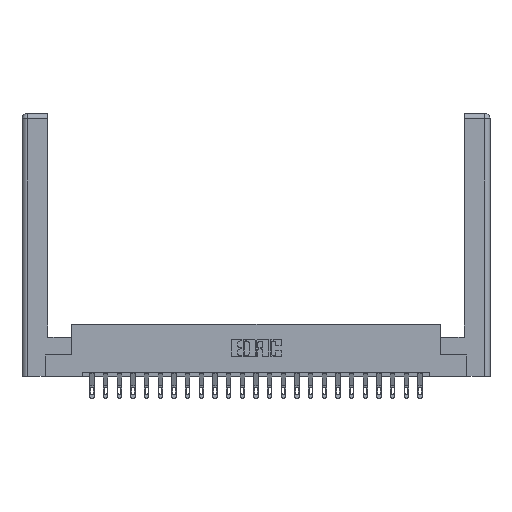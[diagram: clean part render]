
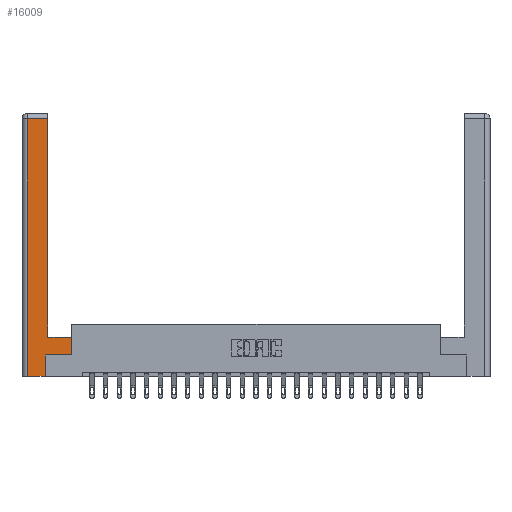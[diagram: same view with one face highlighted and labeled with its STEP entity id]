
A CAD part, top view. The second image highlights one B-rep face of the part: STEP entity #16009.
In plain terms, the highlighted planar face has unit normal (0, 0, 1).
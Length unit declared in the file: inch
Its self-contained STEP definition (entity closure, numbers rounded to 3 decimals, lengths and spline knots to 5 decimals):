
#67 = CARTESIAN_POINT ( 'NONE',  ( 0.0615, 2.94, 0. ) ) ;
#1624 = ORIENTED_EDGE ( 'NONE', *, *, #11793, .T. ) ;
#2462 = CARTESIAN_POINT ( 'NONE',  ( 0.565, 0.45, 0. ) ) ;
#2553 = CARTESIAN_POINT ( 'NONE',  ( 0.0615, 2.94, 0. ) ) ;
#3331 = LINE ( 'NONE', #67, #24392 ) ;
#3742 = CARTESIAN_POINT ( 'NONE',  ( 0.0615, 0., 0. ) ) ;
#4018 = CARTESIAN_POINT ( 'NONE',  ( 0.295, 0.45, 0. ) ) ;
#4036 = DIRECTION ( 'NONE',  ( -1., 0., 0. ) ) ;
#5537 = ORIENTED_EDGE ( 'NONE', *, *, #11222, .T. ) ;
#5653 = EDGE_CURVE ( 'NONE', #11467, #21559, #18575, .T. ) ;
#5938 = LINE ( 'NONE', #4018, #12438 ) ;
#6023 = ORIENTED_EDGE ( 'NONE', *, *, #5653, .T. ) ;
#6710 = DIRECTION ( 'NONE',  ( 0., 0., -1. ) ) ;
#6985 = AXIS2_PLACEMENT_3D ( 'NONE', #17989, #6710, #19988 ) ;
#7150 = FACE_OUTER_BOUND ( 'NONE', #11290, .T. ) ;
#7168 = ORIENTED_EDGE ( 'NONE', *, *, #10393, .T. ) ;
#8019 = PLANE ( 'NONE',  #6985 ) ;
#8891 = DIRECTION ( 'NONE',  ( 1., 0., 0. ) ) ;
#9186 = EDGE_CURVE ( 'NONE', #21559, #15759, #19135, .T. ) ;
#9384 = ORIENTED_EDGE ( 'NONE', *, *, #10762, .T. ) ;
#9606 = LINE ( 'NONE', #22408, #11954 ) ;
#10129 = LINE ( 'NONE', #16510, #13332 ) ;
#10307 = DIRECTION ( 'NONE',  ( 0., 1., 0. ) ) ;
#10378 = VERTEX_POINT ( 'NONE', #18408 ) ;
#10393 = EDGE_CURVE ( 'NONE', #10378, #23335, #9606, .T. ) ;
#10488 = VECTOR ( 'NONE', #10307, 39.37008 ) ;
#10699 = CARTESIAN_POINT ( 'NONE',  ( 0.265, 0.245, 0. ) ) ;
#10762 = EDGE_CURVE ( 'NONE', #22524, #22475, #18768, .T. ) ;
#11222 = EDGE_CURVE ( 'NONE', #22475, #11467, #3331, .T. ) ;
#11290 = EDGE_LOOP ( 'NONE', ( #9384, #5537, #6023, #20501, #12823, #7168, #1624, #17754 ) ) ;
#11429 = CARTESIAN_POINT ( 'NONE',  ( 0.565, 0.245, 0. ) ) ;
#11467 = VERTEX_POINT ( 'NONE', #2553 ) ;
#11793 = EDGE_CURVE ( 'NONE', #23335, #22470, #10129, .T. ) ;
#11954 = VECTOR ( 'NONE', #8891, 39.37008 ) ;
#12438 = VECTOR ( 'NONE', #17235, 39.37008 ) ;
#12600 = VECTOR ( 'NONE', #14992, 39.37008 ) ;
#12648 = CARTESIAN_POINT ( 'NONE',  ( 0.265, 0., 0. ) ) ;
#12650 = DIRECTION ( 'NONE',  ( 0., 1., 0. ) ) ;
#12823 = ORIENTED_EDGE ( 'NONE', *, *, #22103, .T. ) ;
#13332 = VECTOR ( 'NONE', #20247, 39.37008 ) ;
#14992 = DIRECTION ( 'NONE',  ( 1., 0., 0. ) ) ;
#15474 = CARTESIAN_POINT ( 'NONE',  ( 0.295, 2.94, 0. ) ) ;
#15759 = VERTEX_POINT ( 'NONE', #12648 ) ;
#16009 = ADVANCED_FACE ( 'NONE', ( #7150 ), #8019, .F. ) ;
#16239 = VECTOR ( 'NONE', #12650, 39.37008 ) ;
#16510 = CARTESIAN_POINT ( 'NONE',  ( 0.565, 0.45, 0. ) ) ;
#17193 = CARTESIAN_POINT ( 'NONE',  ( 0.0615, 0., 0. ) ) ;
#17235 = DIRECTION ( 'NONE',  ( -1., 0., 0. ) ) ;
#17298 = EDGE_CURVE ( 'NONE', #22470, #22524, #5938, .T. ) ;
#17525 = CARTESIAN_POINT ( 'NONE',  ( 0.295, 0.45, 0. ) ) ;
#17754 = ORIENTED_EDGE ( 'NONE', *, *, #17298, .T. ) ;
#17989 = CARTESIAN_POINT ( 'NONE',  ( 0., 0., 0. ) ) ;
#18408 = CARTESIAN_POINT ( 'NONE',  ( 0.265, 0.245, 0. ) ) ;
#18575 = LINE ( 'NONE', #3742, #21258 ) ;
#18768 = LINE ( 'NONE', #19250, #10488 ) ;
#19135 = LINE ( 'NONE', #22499, #12600 ) ;
#19250 = CARTESIAN_POINT ( 'NONE',  ( 0.295, 3., 0. ) ) ;
#19988 = DIRECTION ( 'NONE',  ( -1., 0., 0. ) ) ;
#20104 = LINE ( 'NONE', #10699, #16239 ) ;
#20247 = DIRECTION ( 'NONE',  ( 0., 1., 0. ) ) ;
#20501 = ORIENTED_EDGE ( 'NONE', *, *, #9186, .T. ) ;
#20566 = DIRECTION ( 'NONE',  ( 0., -1., 0. ) ) ;
#21258 = VECTOR ( 'NONE', #20566, 39.37008 ) ;
#21559 = VERTEX_POINT ( 'NONE', #17193 ) ;
#22103 = EDGE_CURVE ( 'NONE', #15759, #10378, #20104, .T. ) ;
#22408 = CARTESIAN_POINT ( 'NONE',  ( 0.565, 0.245, 0. ) ) ;
#22470 = VERTEX_POINT ( 'NONE', #2462 ) ;
#22475 = VERTEX_POINT ( 'NONE', #15474 ) ;
#22499 = CARTESIAN_POINT ( 'NONE',  ( 0.265, 0., 0. ) ) ;
#22524 = VERTEX_POINT ( 'NONE', #17525 ) ;
#23335 = VERTEX_POINT ( 'NONE', #11429 ) ;
#24392 = VECTOR ( 'NONE', #4036, 39.37008 ) ;
